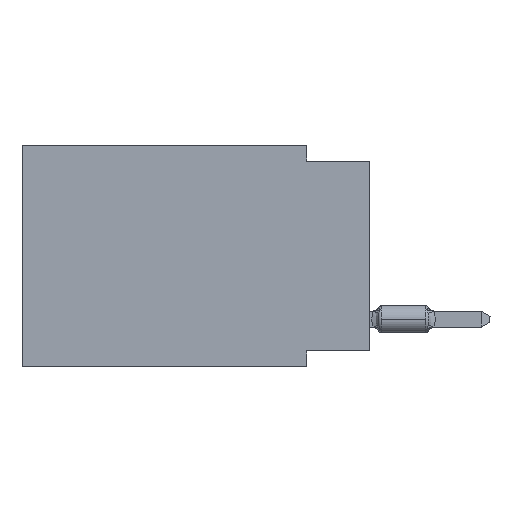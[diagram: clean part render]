
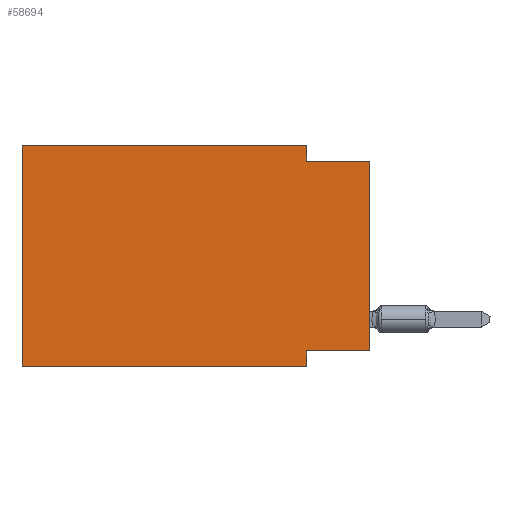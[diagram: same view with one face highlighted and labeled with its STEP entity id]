
A CAD part, left-side view. The second image highlights one B-rep face of the part: STEP entity #58694.
In plain terms, the highlighted planar face has unit normal (-1, 0, 0).
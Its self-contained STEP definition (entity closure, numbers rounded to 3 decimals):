
#241 = VERTEX_POINT ( 'NONE', #50461 ) ;
#1550 = EDGE_CURVE ( 'NONE', #57376, #40653, #61368, .T. ) ;
#3392 = LINE ( 'NONE', #59211, #77835 ) ;
#7454 = DIRECTION ( 'NONE',  ( 0., 0., -1. ) ) ;
#7814 = EDGE_CURVE ( 'NONE', #49029, #83522, #16994, .T. ) ;
#8297 = DIRECTION ( 'NONE',  ( 1., 0., 0. ) ) ;
#11187 = CARTESIAN_POINT ( 'NONE',  ( 0., 2.54, 0. ) ) ;
#11989 = VERTEX_POINT ( 'NONE', #38270 ) ;
#12118 = VECTOR ( 'NONE', #73083, 1000. ) ;
#12977 = LINE ( 'NONE', #34557, #23808 ) ;
#13747 = LINE ( 'NONE', #69110, #47116 ) ;
#15492 = EDGE_LOOP ( 'NONE', ( #85782, #21963, #79154, #39398, #64991, #85489, #60501, #45427 ) ) ;
#16991 = DIRECTION ( 'NONE',  ( 0., 1., 0. ) ) ;
#16994 = LINE ( 'NONE', #71476, #73096 ) ;
#18517 = CARTESIAN_POINT ( 'NONE',  ( 0., 2.54, -8.89 ) ) ;
#20322 = EDGE_CURVE ( 'NONE', #57376, #11989, #12977, .T. ) ;
#20904 = DIRECTION ( 'NONE',  ( 0., -1., 0. ) ) ;
#21963 = ORIENTED_EDGE ( 'NONE', *, *, #54495, .F. ) ;
#22134 = CARTESIAN_POINT ( 'NONE',  ( 0., 0., -8.255 ) ) ;
#23808 = VECTOR ( 'NONE', #81849, 1000. ) ;
#25566 = CARTESIAN_POINT ( 'NONE',  ( 0., 2.54, -8.255 ) ) ;
#29341 = CARTESIAN_POINT ( 'NONE',  ( 0., 0., -0.635 ) ) ;
#30824 = DIRECTION ( 'NONE',  ( 0., -1., 0. ) ) ;
#30914 = VECTOR ( 'NONE', #16991, 1000. ) ;
#33895 = CARTESIAN_POINT ( 'NONE',  ( 0., 13.97, 0. ) ) ;
#34557 = CARTESIAN_POINT ( 'NONE',  ( 0., 13.97, -8.89 ) ) ;
#35944 = LINE ( 'NONE', #36810, #30914 ) ;
#36810 = CARTESIAN_POINT ( 'NONE',  ( 0., 0., -8.255 ) ) ;
#36989 = EDGE_CURVE ( 'NONE', #40653, #73413, #3392, .T. ) ;
#38270 = CARTESIAN_POINT ( 'NONE',  ( 0., 2.54, -8.89 ) ) ;
#38340 = EDGE_CURVE ( 'NONE', #73547, #11989, #52720, .T. ) ;
#39398 = ORIENTED_EDGE ( 'NONE', *, *, #36989, .F. ) ;
#40498 = CARTESIAN_POINT ( 'NONE',  ( 0., 13.97, 0. ) ) ;
#40653 = VERTEX_POINT ( 'NONE', #40498 ) ;
#42007 = EDGE_CURVE ( 'NONE', #49029, #73547, #35944, .T. ) ;
#45427 = ORIENTED_EDGE ( 'NONE', *, *, #42007, .F. ) ;
#47116 = VECTOR ( 'NONE', #7454, 1000. ) ;
#48368 = FACE_OUTER_BOUND ( 'NONE', #15492, .T. ) ;
#49029 = VERTEX_POINT ( 'NONE', #22134 ) ;
#50001 = AXIS2_PLACEMENT_3D ( 'NONE', #57332, #8297, #75825 ) ;
#50461 = CARTESIAN_POINT ( 'NONE',  ( 0., 2.54, -0.635 ) ) ;
#52720 = LINE ( 'NONE', #18517, #82103 ) ;
#52783 = EDGE_CURVE ( 'NONE', #73413, #241, #13747, .T. ) ;
#53627 = DIRECTION ( 'NONE',  ( 0., 0., -1. ) ) ;
#54495 = EDGE_CURVE ( 'NONE', #241, #83522, #63214, .T. ) ;
#57332 = CARTESIAN_POINT ( 'NONE',  ( 0., 13.97, 0. ) ) ;
#57376 = VERTEX_POINT ( 'NONE', #75790 ) ;
#58694 = ADVANCED_FACE ( 'NONE', ( #48368 ), #64077, .F. ) ;
#59211 = CARTESIAN_POINT ( 'NONE',  ( 0., 13.97, 0. ) ) ;
#60501 = ORIENTED_EDGE ( 'NONE', *, *, #38340, .F. ) ;
#61368 = LINE ( 'NONE', #33895, #12118 ) ;
#61718 = VECTOR ( 'NONE', #20904, 1000. ) ;
#63214 = LINE ( 'NONE', #75830, #61718 ) ;
#64077 = PLANE ( 'NONE',  #50001 ) ;
#64991 = ORIENTED_EDGE ( 'NONE', *, *, #1550, .F. ) ;
#66057 = DIRECTION ( 'NONE',  ( 0., 0., 1. ) ) ;
#69110 = CARTESIAN_POINT ( 'NONE',  ( 0., 2.54, 0. ) ) ;
#71476 = CARTESIAN_POINT ( 'NONE',  ( 0., 0., 0. ) ) ;
#73083 = DIRECTION ( 'NONE',  ( 0., 0., 1. ) ) ;
#73096 = VECTOR ( 'NONE', #66057, 1000. ) ;
#73413 = VERTEX_POINT ( 'NONE', #11187 ) ;
#73547 = VERTEX_POINT ( 'NONE', #25566 ) ;
#75790 = CARTESIAN_POINT ( 'NONE',  ( 0., 13.97, -8.89 ) ) ;
#75825 = DIRECTION ( 'NONE',  ( 0., 0., -1. ) ) ;
#75830 = CARTESIAN_POINT ( 'NONE',  ( 0., 0., -0.635 ) ) ;
#77835 = VECTOR ( 'NONE', #30824, 1000. ) ;
#79154 = ORIENTED_EDGE ( 'NONE', *, *, #52783, .F. ) ;
#81849 = DIRECTION ( 'NONE',  ( 0., -1., 0. ) ) ;
#82103 = VECTOR ( 'NONE', #53627, 1000. ) ;
#83522 = VERTEX_POINT ( 'NONE', #29341 ) ;
#85489 = ORIENTED_EDGE ( 'NONE', *, *, #20322, .T. ) ;
#85782 = ORIENTED_EDGE ( 'NONE', *, *, #7814, .T. ) ;
